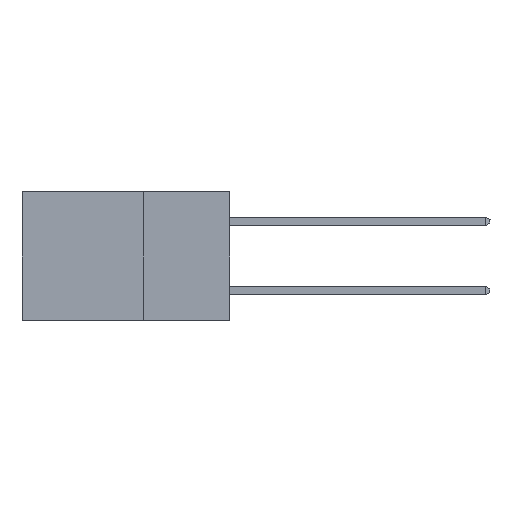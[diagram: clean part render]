
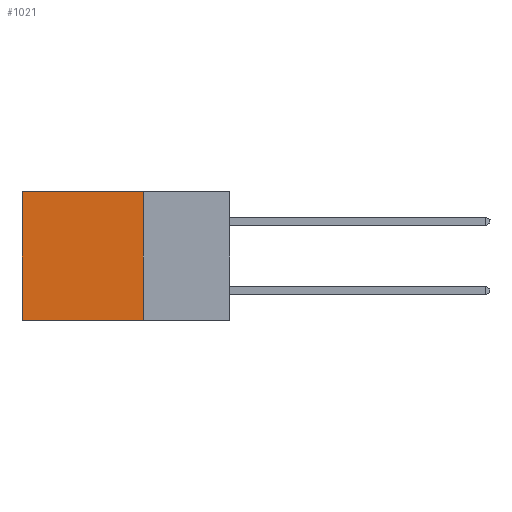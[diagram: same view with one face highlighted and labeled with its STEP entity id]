
A CAD part, left-side view. The second image highlights one B-rep face of the part: STEP entity #1021.
In plain terms, the highlighted planar face has unit normal (-1, 0, 0).
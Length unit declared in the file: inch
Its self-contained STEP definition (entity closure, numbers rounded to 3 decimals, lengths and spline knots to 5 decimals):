
#63 = VECTOR ( 'NONE', #8010, 39.37008 ) ;
#439 = CARTESIAN_POINT ( 'NONE',  ( 0.2615, 0.25, -0.37 ) ) ;
#457 = DIRECTION ( 'NONE',  ( 0., 0., -1. ) ) ;
#527 = LINE ( 'NONE', #3780, #63 ) ;
#631 = VECTOR ( 'NONE', #6227, 39.37008 ) ;
#1021 = ADVANCED_FACE ( 'NONE', ( #9877 ), #13056, .F. ) ;
#1307 = DIRECTION ( 'NONE',  ( 0., 0., -1. ) ) ;
#1373 = LINE ( 'NONE', #2345, #5783 ) ;
#1495 = LINE ( 'NONE', #4744, #11925 ) ;
#2345 = CARTESIAN_POINT ( 'NONE',  ( 0.2615, 0.6, -0.37 ) ) ;
#2351 = CARTESIAN_POINT ( 'NONE',  ( 0.2615, 0.6, -0.37 ) ) ;
#3042 = CARTESIAN_POINT ( 'NONE',  ( 0.2615, 0.25, 0. ) ) ;
#3207 = AXIS2_PLACEMENT_3D ( 'NONE', #439, #9817, #3561 ) ;
#3458 = EDGE_CURVE ( 'NONE', #12727, #10884, #11504, .T. ) ;
#3561 = DIRECTION ( 'NONE',  ( 0., 0., -1. ) ) ;
#3780 = CARTESIAN_POINT ( 'NONE',  ( 0.2615, 0.25, -0.37 ) ) ;
#4501 = EDGE_CURVE ( 'NONE', #12727, #10963, #1495, .T. ) ;
#4700 = CARTESIAN_POINT ( 'NONE',  ( 0.2615, 0.25, 0. ) ) ;
#4744 = CARTESIAN_POINT ( 'NONE',  ( 0.2615, 0.25, -0.37 ) ) ;
#5277 = ORIENTED_EDGE ( 'NONE', *, *, #4501, .F. ) ;
#5783 = VECTOR ( 'NONE', #1307, 39.37008 ) ;
#6227 = DIRECTION ( 'NONE',  ( 0., 1., 0. ) ) ;
#6634 = ORIENTED_EDGE ( 'NONE', *, *, #3458, .T. ) ;
#8010 = DIRECTION ( 'NONE',  ( 0., 1., 0. ) ) ;
#8477 = EDGE_CURVE ( 'NONE', #10963, #11538, #527, .T. ) ;
#8911 = ORIENTED_EDGE ( 'NONE', *, *, #8477, .F. ) ;
#9504 = ORIENTED_EDGE ( 'NONE', *, *, #9585, .T. ) ;
#9585 = EDGE_CURVE ( 'NONE', #10884, #11538, #1373, .T. ) ;
#9790 = CARTESIAN_POINT ( 'NONE',  ( 0.2615, 0.25, -0.37 ) ) ;
#9817 = DIRECTION ( 'NONE',  ( 1., 0., 0. ) ) ;
#9877 = FACE_OUTER_BOUND ( 'NONE', #10791, .T. ) ;
#10791 = EDGE_LOOP ( 'NONE', ( #9504, #8911, #5277, #6634 ) ) ;
#10884 = VERTEX_POINT ( 'NONE', #11380 ) ;
#10963 = VERTEX_POINT ( 'NONE', #9790 ) ;
#11380 = CARTESIAN_POINT ( 'NONE',  ( 0.2615, 0.6, 0. ) ) ;
#11504 = LINE ( 'NONE', #3042, #631 ) ;
#11538 = VERTEX_POINT ( 'NONE', #2351 ) ;
#11925 = VECTOR ( 'NONE', #457, 39.37008 ) ;
#12727 = VERTEX_POINT ( 'NONE', #4700 ) ;
#13056 = PLANE ( 'NONE',  #3207 ) ;
